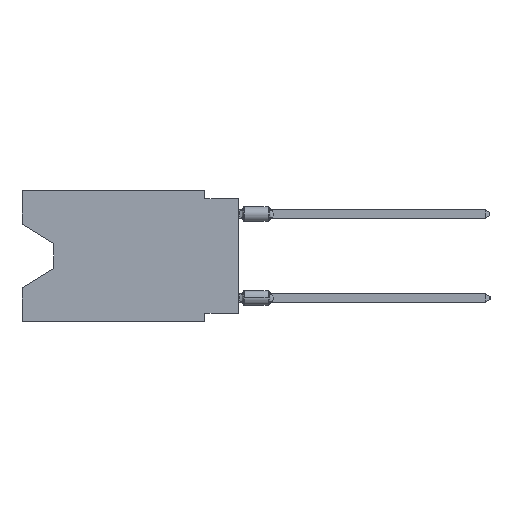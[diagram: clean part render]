
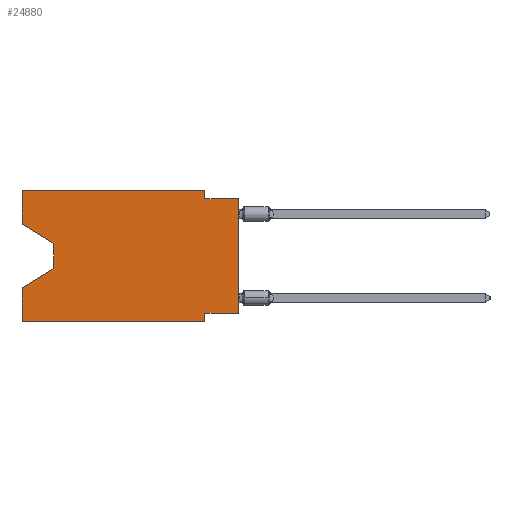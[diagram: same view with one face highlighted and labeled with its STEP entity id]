
A CAD part, left-side view. The second image highlights one B-rep face of the part: STEP entity #24880.
In plain terms, the highlighted planar face has unit normal (-1, 0, 0).
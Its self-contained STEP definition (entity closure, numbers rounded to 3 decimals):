
#362 = CARTESIAN_POINT ( 'NONE',  ( 0., 13.97, -4.013 ) ) ;
#1912 = DIRECTION ( 'NONE',  ( 0., -1., 0. ) ) ;
#2541 = AXIS2_PLACEMENT_3D ( 'NONE', #44509, #52916, #24412 ) ;
#3006 = PLANE ( 'NONE',  #2541 ) ;
#3067 = CARTESIAN_POINT ( 'NONE',  ( 0., 2.54, -9.906 ) ) ;
#3331 = DIRECTION ( 'NONE',  ( 0., 0.855, -0.519 ) ) ;
#3544 = LINE ( 'NONE', #24952, #13657 ) ;
#3724 = DIRECTION ( 'NONE',  ( 0., 0., -1. ) ) ;
#3804 = DIRECTION ( 'NONE',  ( 0., 0., 1. ) ) ;
#4410 = VECTOR ( 'NONE', #39431, 1000. ) ;
#4588 = ORIENTED_EDGE ( 'NONE', *, *, #11425, .T. ) ;
#5780 = ORIENTED_EDGE ( 'NONE', *, *, #10569, .T. ) ;
#6688 = EDGE_CURVE ( 'NONE', #32687, #33052, #39162, .T. ) ;
#7669 = LINE ( 'NONE', #15290, #45503 ) ;
#7873 = VECTOR ( 'NONE', #40860, 1000. ) ;
#8062 = LINE ( 'NONE', #12407, #48125 ) ;
#8433 = VERTEX_POINT ( 'NONE', #36968 ) ;
#10569 = EDGE_CURVE ( 'NONE', #8433, #24066, #42251, .T. ) ;
#11033 = VECTOR ( 'NONE', #28808, 1000. ) ;
#11306 = EDGE_CURVE ( 'NONE', #19227, #24066, #47054, .T. ) ;
#11425 = EDGE_CURVE ( 'NONE', #36090, #23674, #7669, .T. ) ;
#12232 = ORIENTED_EDGE ( 'NONE', *, *, #16036, .F. ) ;
#12407 = CARTESIAN_POINT ( 'NONE',  ( 0., 2.54, 0. ) ) ;
#12894 = EDGE_CURVE ( 'NONE', #31988, #30485, #16416, .T. ) ;
#13657 = VECTOR ( 'NONE', #3804, 1000. ) ;
#14614 = CARTESIAN_POINT ( 'NONE',  ( 0., 2.54, 0. ) ) ;
#14713 = LINE ( 'NONE', #27435, #31079 ) ;
#15290 = CARTESIAN_POINT ( 'NONE',  ( 0., 13.97, -5.893 ) ) ;
#15943 = VERTEX_POINT ( 'NONE', #33381 ) ;
#16036 = EDGE_CURVE ( 'NONE', #32687, #31988, #35264, .T. ) ;
#16416 = LINE ( 'NONE', #49247, #7873 ) ;
#16815 = VECTOR ( 'NONE', #47139, 1000. ) ;
#17992 = LINE ( 'NONE', #362, #24563 ) ;
#18271 = ORIENTED_EDGE ( 'NONE', *, *, #6688, .T. ) ;
#18823 = ORIENTED_EDGE ( 'NONE', *, *, #11306, .F. ) ;
#19007 = LINE ( 'NONE', #52624, #44074 ) ;
#19227 = VERTEX_POINT ( 'NONE', #46146 ) ;
#20623 = CARTESIAN_POINT ( 'NONE',  ( 0., 13.97, -4.013 ) ) ;
#21234 = VECTOR ( 'NONE', #43514, 1000. ) ;
#22234 = CARTESIAN_POINT ( 'NONE',  ( 0., 16.383, 0. ) ) ;
#22956 = CARTESIAN_POINT ( 'NONE',  ( 0., 2.54, -9.271 ) ) ;
#23674 = VERTEX_POINT ( 'NONE', #44761 ) ;
#24066 = VERTEX_POINT ( 'NONE', #48707 ) ;
#24247 = ORIENTED_EDGE ( 'NONE', *, *, #30247, .F. ) ;
#24412 = DIRECTION ( 'NONE',  ( 0., 0., -1. ) ) ;
#24563 = VECTOR ( 'NONE', #37808, 1000. ) ;
#24880 = ADVANCED_FACE ( 'NONE', ( #28218 ), #3006, .F. ) ;
#24952 = CARTESIAN_POINT ( 'NONE',  ( 0., 16.383, 0. ) ) ;
#27064 = EDGE_CURVE ( 'NONE', #47559, #15943, #45617, .T. ) ;
#27104 = DIRECTION ( 'NONE',  ( 0., 0., 1. ) ) ;
#27141 = CARTESIAN_POINT ( 'NONE',  ( 0., 13.97, -5.893 ) ) ;
#27435 = CARTESIAN_POINT ( 'NONE',  ( 0., 0., -9.271 ) ) ;
#27618 = CARTESIAN_POINT ( 'NONE',  ( 0., 16.383, 0. ) ) ;
#28218 = FACE_OUTER_BOUND ( 'NONE', #43498, .T. ) ;
#28808 = DIRECTION ( 'NONE',  ( 0., 0., -1. ) ) ;
#29773 = CARTESIAN_POINT ( 'NONE',  ( 0., 0., 0. ) ) ;
#30247 = EDGE_CURVE ( 'NONE', #8433, #47559, #14713, .T. ) ;
#30485 = VERTEX_POINT ( 'NONE', #14614 ) ;
#31018 = CARTESIAN_POINT ( 'NONE',  ( 0., 16.383, -2.546 ) ) ;
#31079 = VECTOR ( 'NONE', #35598, 1000. ) ;
#31988 = VERTEX_POINT ( 'NONE', #27618 ) ;
#32687 = VERTEX_POINT ( 'NONE', #42102 ) ;
#33052 = VERTEX_POINT ( 'NONE', #20623 ) ;
#33381 = CARTESIAN_POINT ( 'NONE',  ( 0., 2.54, -9.906 ) ) ;
#35125 = CARTESIAN_POINT ( 'NONE',  ( 0., 0., -0.635 ) ) ;
#35264 = LINE ( 'NONE', #22234, #42654 ) ;
#35598 = DIRECTION ( 'NONE',  ( 0., 1., 0. ) ) ;
#36090 = VERTEX_POINT ( 'NONE', #27141 ) ;
#36673 = ORIENTED_EDGE ( 'NONE', *, *, #45236, .T. ) ;
#36870 = VERTEX_POINT ( 'NONE', #47641 ) ;
#36968 = CARTESIAN_POINT ( 'NONE',  ( 0., 0., -9.271 ) ) ;
#37243 = ORIENTED_EDGE ( 'NONE', *, *, #49779, .F. ) ;
#37808 = DIRECTION ( 'NONE',  ( 0., 0., -1. ) ) ;
#39162 = LINE ( 'NONE', #31018, #4410 ) ;
#39431 = DIRECTION ( 'NONE',  ( 0., -0.855, -0.519 ) ) ;
#39839 = ORIENTED_EDGE ( 'NONE', *, *, #47348, .F. ) ;
#40860 = DIRECTION ( 'NONE',  ( 0., -1., 0. ) ) ;
#42102 = CARTESIAN_POINT ( 'NONE',  ( 0., 16.383, -2.546 ) ) ;
#42251 = LINE ( 'NONE', #29773, #16815 ) ;
#42654 = VECTOR ( 'NONE', #27104, 1000. ) ;
#43364 = ORIENTED_EDGE ( 'NONE', *, *, #27064, .F. ) ;
#43498 = EDGE_LOOP ( 'NONE', ( #18271, #36673, #4588, #37243, #53297, #43364, #24247, #5780, #18823, #39839, #50959, #12232 ) ) ;
#43514 = DIRECTION ( 'NONE',  ( 0., -1., 0. ) ) ;
#44074 = VECTOR ( 'NONE', #1912, 1000. ) ;
#44509 = CARTESIAN_POINT ( 'NONE',  ( 0., 16.383, 0. ) ) ;
#44761 = CARTESIAN_POINT ( 'NONE',  ( 0., 16.383, -7.36 ) ) ;
#45236 = EDGE_CURVE ( 'NONE', #33052, #36090, #17992, .T. ) ;
#45503 = VECTOR ( 'NONE', #3331, 1000. ) ;
#45617 = LINE ( 'NONE', #3067, #11033 ) ;
#46146 = CARTESIAN_POINT ( 'NONE',  ( 0., 2.54, -0.635 ) ) ;
#47054 = LINE ( 'NONE', #35125, #21234 ) ;
#47139 = DIRECTION ( 'NONE',  ( 0., 0., 1. ) ) ;
#47348 = EDGE_CURVE ( 'NONE', #30485, #19227, #8062, .T. ) ;
#47559 = VERTEX_POINT ( 'NONE', #22956 ) ;
#47641 = CARTESIAN_POINT ( 'NONE',  ( 0., 16.383, -9.906 ) ) ;
#48125 = VECTOR ( 'NONE', #3724, 1000. ) ;
#48707 = CARTESIAN_POINT ( 'NONE',  ( 0., 0., -0.635 ) ) ;
#49247 = CARTESIAN_POINT ( 'NONE',  ( 0., 16.383, 0. ) ) ;
#49779 = EDGE_CURVE ( 'NONE', #36870, #23674, #3544, .T. ) ;
#50959 = ORIENTED_EDGE ( 'NONE', *, *, #12894, .F. ) ;
#52624 = CARTESIAN_POINT ( 'NONE',  ( 0., 16.383, -9.906 ) ) ;
#52916 = DIRECTION ( 'NONE',  ( 1., 0., 0. ) ) ;
#53083 = EDGE_CURVE ( 'NONE', #36870, #15943, #19007, .T. ) ;
#53297 = ORIENTED_EDGE ( 'NONE', *, *, #53083, .T. ) ;
